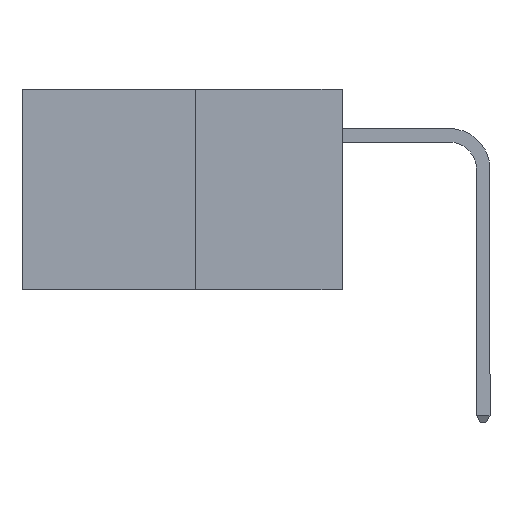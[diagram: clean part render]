
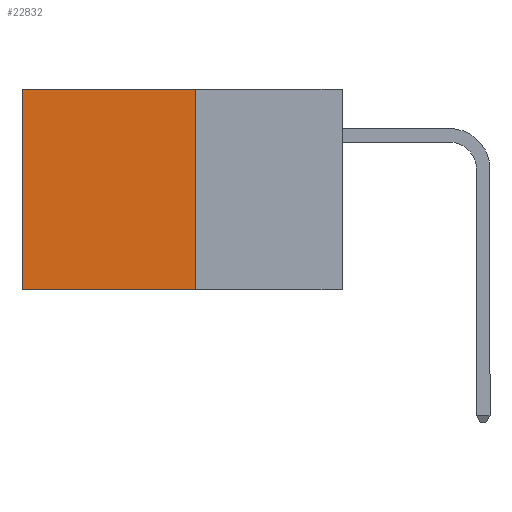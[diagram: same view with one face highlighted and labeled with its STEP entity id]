
A CAD part, left-side view. The second image highlights one B-rep face of the part: STEP entity #22832.
In plain terms, the highlighted planar face has unit normal (-1, 0, 0).
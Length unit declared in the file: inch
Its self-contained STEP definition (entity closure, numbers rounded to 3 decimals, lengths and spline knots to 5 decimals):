
#2274 = CARTESIAN_POINT ( 'NONE',  ( 0.277, 0.59, -0.37 ) ) ;
#2991 = CARTESIAN_POINT ( 'NONE',  ( 0.277, 0.27, 0. ) ) ;
#3668 = CARTESIAN_POINT ( 'NONE',  ( 0.277, 0.27, -0.37 ) ) ;
#3717 = ORIENTED_EDGE ( 'NONE', *, *, #15667, .T. ) ;
#3733 = LINE ( 'NONE', #10656, #14371 ) ;
#3840 = LINE ( 'NONE', #9573, #5212 ) ;
#4187 = EDGE_CURVE ( 'NONE', #14332, #19948, #6412, .T. ) ;
#5212 = VECTOR ( 'NONE', #15876, 39.37008 ) ;
#5490 = CARTESIAN_POINT ( 'NONE',  ( 0.277, 0.27, -0.37 ) ) ;
#5589 = DIRECTION ( 'NONE',  ( 0., 0., -1. ) ) ;
#6412 = LINE ( 'NONE', #5490, #18272 ) ;
#7867 = DIRECTION ( 'NONE',  ( 0., 0., -1. ) ) ;
#8922 = AXIS2_PLACEMENT_3D ( 'NONE', #9907, #20435, #7867 ) ;
#9573 = CARTESIAN_POINT ( 'NONE',  ( 0.277, 0.59, -0.37 ) ) ;
#9881 = CARTESIAN_POINT ( 'NONE',  ( 0.277, 0.27, 0. ) ) ;
#9907 = CARTESIAN_POINT ( 'NONE',  ( 0.277, 0.27, -0.37 ) ) ;
#10198 = VERTEX_POINT ( 'NONE', #10933 ) ;
#10656 = CARTESIAN_POINT ( 'NONE',  ( 0.277, 0.27, -0.37 ) ) ;
#10933 = CARTESIAN_POINT ( 'NONE',  ( 0.277, 0.59, 0. ) ) ;
#13178 = FACE_OUTER_BOUND ( 'NONE', #25339, .T. ) ;
#13933 = VECTOR ( 'NONE', #16178, 39.37008 ) ;
#13985 = ORIENTED_EDGE ( 'NONE', *, *, #4187, .F. ) ;
#14332 = VERTEX_POINT ( 'NONE', #2991 ) ;
#14371 = VECTOR ( 'NONE', #25200, 39.37008 ) ;
#15667 = EDGE_CURVE ( 'NONE', #10198, #25976, #3840, .T. ) ;
#15876 = DIRECTION ( 'NONE',  ( 0., 0., -1. ) ) ;
#16178 = DIRECTION ( 'NONE',  ( 0., 1., 0. ) ) ;
#17311 = EDGE_CURVE ( 'NONE', #19948, #25976, #3733, .T. ) ;
#18272 = VECTOR ( 'NONE', #5589, 39.37008 ) ;
#19948 = VERTEX_POINT ( 'NONE', #3668 ) ;
#20128 = LINE ( 'NONE', #9881, #13933 ) ;
#20435 = DIRECTION ( 'NONE',  ( 1., 0., 0. ) ) ;
#21549 = EDGE_CURVE ( 'NONE', #14332, #10198, #20128, .T. ) ;
#22832 = ADVANCED_FACE ( 'NONE', ( #13178 ), #24477, .F. ) ;
#24477 = PLANE ( 'NONE',  #8922 ) ;
#25192 = ORIENTED_EDGE ( 'NONE', *, *, #17311, .F. ) ;
#25200 = DIRECTION ( 'NONE',  ( 0., 1., 0. ) ) ;
#25339 = EDGE_LOOP ( 'NONE', ( #3717, #25192, #13985, #26475 ) ) ;
#25976 = VERTEX_POINT ( 'NONE', #2274 ) ;
#26475 = ORIENTED_EDGE ( 'NONE', *, *, #21549, .T. ) ;
